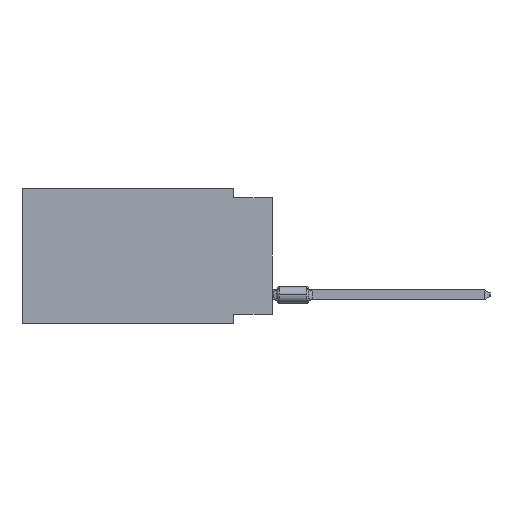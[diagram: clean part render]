
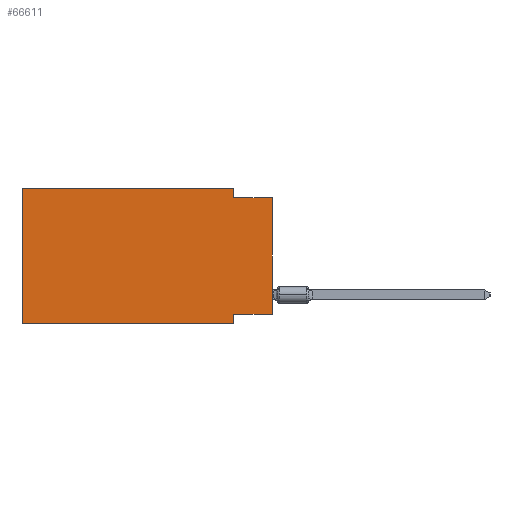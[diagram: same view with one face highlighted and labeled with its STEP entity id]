
A CAD part, left-side view. The second image highlights one B-rep face of the part: STEP entity #66611.
In plain terms, the highlighted planar face has unit normal (-1, 0, 0).
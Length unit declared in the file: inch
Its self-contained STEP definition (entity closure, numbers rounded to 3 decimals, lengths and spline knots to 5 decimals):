
#1990 = ORIENTED_EDGE ( 'NONE', *, *, #16436, .F. ) ;
#2873 = VERTEX_POINT ( 'NONE', #19491 ) ;
#4245 = LINE ( 'NONE', #48958, #18061 ) ;
#5414 = LINE ( 'NONE', #41989, #42734 ) ;
#5674 = CARTESIAN_POINT ( 'NONE',  ( 0., 0.1, -0.025 ) ) ;
#6859 = CARTESIAN_POINT ( 'NONE',  ( 0., 0.1, 0. ) ) ;
#7140 = VERTEX_POINT ( 'NONE', #83503 ) ;
#9085 = ORIENTED_EDGE ( 'NONE', *, *, #21617, .F. ) ;
#9833 = DIRECTION ( 'NONE',  ( 0., 1., 0. ) ) ;
#13986 = DIRECTION ( 'NONE',  ( 1., 0., 0. ) ) ;
#14688 = ORIENTED_EDGE ( 'NONE', *, *, #93546, .T. ) ;
#14752 = VERTEX_POINT ( 'NONE', #37182 ) ;
#15377 = LINE ( 'NONE', #66838, #82319 ) ;
#15677 = CARTESIAN_POINT ( 'NONE',  ( 0., 0., 0. ) ) ;
#16152 = DIRECTION ( 'NONE',  ( 0., 0., 1. ) ) ;
#16298 = VERTEX_POINT ( 'NONE', #43787 ) ;
#16436 = EDGE_CURVE ( 'NONE', #61065, #7140, #15377, .T. ) ;
#18061 = VECTOR ( 'NONE', #71080, 39.37008 ) ;
#19491 = CARTESIAN_POINT ( 'NONE',  ( 0., 0.1, -0.325 ) ) ;
#20256 = VECTOR ( 'NONE', #64571, 39.37008 ) ;
#21617 = EDGE_CURVE ( 'NONE', #7140, #92543, #91471, .T. ) ;
#22892 = LINE ( 'NONE', #15677, #34242 ) ;
#23430 = ORIENTED_EDGE ( 'NONE', *, *, #23758, .F. ) ;
#23758 = EDGE_CURVE ( 'NONE', #2873, #38565, #5414, .T. ) ;
#24232 = VECTOR ( 'NONE', #55381, 39.37008 ) ;
#25238 = LINE ( 'NONE', #89677, #42904 ) ;
#25363 = LINE ( 'NONE', #68623, #52701 ) ;
#29501 = EDGE_CURVE ( 'NONE', #92543, #34889, #35250, .T. ) ;
#34242 = VECTOR ( 'NONE', #16152, 39.37008 ) ;
#34720 = EDGE_CURVE ( 'NONE', #61065, #38565, #4245, .T. ) ;
#34889 = VERTEX_POINT ( 'NONE', #5674 ) ;
#34916 = ORIENTED_EDGE ( 'NONE', *, *, #93664, .F. ) ;
#35250 = LINE ( 'NONE', #6859, #20256 ) ;
#37182 = CARTESIAN_POINT ( 'NONE',  ( 0., 0., -0.325 ) ) ;
#38341 = ORIENTED_EDGE ( 'NONE', *, *, #38486, .F. ) ;
#38486 = EDGE_CURVE ( 'NONE', #14752, #2873, #25238, .T. ) ;
#38565 = VERTEX_POINT ( 'NONE', #92508 ) ;
#41989 = CARTESIAN_POINT ( 'NONE',  ( 0., 0.1, -0.35 ) ) ;
#42734 = VECTOR ( 'NONE', #71293, 39.37008 ) ;
#42904 = VECTOR ( 'NONE', #9833, 39.37008 ) ;
#43349 = DIRECTION ( 'NONE',  ( 0., 0., -1. ) ) ;
#43787 = CARTESIAN_POINT ( 'NONE',  ( 0., 0., -0.025 ) ) ;
#45525 = CARTESIAN_POINT ( 'NONE',  ( 0., 0.1, 0. ) ) ;
#48652 = CARTESIAN_POINT ( 'NONE',  ( 0., 0.645, 0. ) ) ;
#48958 = CARTESIAN_POINT ( 'NONE',  ( 0., 0.645, -0.35 ) ) ;
#52701 = VECTOR ( 'NONE', #90287, 39.37008 ) ;
#55381 = DIRECTION ( 'NONE',  ( 0., -1., 0. ) ) ;
#56013 = CARTESIAN_POINT ( 'NONE',  ( 0., 0.645, -0.35 ) ) ;
#59026 = EDGE_LOOP ( 'NONE', ( #14688, #34916, #84128, #9085, #1990, #85969, #23430, #38341 ) ) ;
#61065 = VERTEX_POINT ( 'NONE', #56013 ) ;
#64571 = DIRECTION ( 'NONE',  ( 0., 0., -1. ) ) ;
#65890 = DIRECTION ( 'NONE',  ( 0., 0., 1. ) ) ;
#66611 = ADVANCED_FACE ( 'NONE', ( #73586 ), #73121, .F. ) ;
#66838 = CARTESIAN_POINT ( 'NONE',  ( 0., 0.645, 0. ) ) ;
#68424 = AXIS2_PLACEMENT_3D ( 'NONE', #86619, #13986, #43349 ) ;
#68623 = CARTESIAN_POINT ( 'NONE',  ( 0., 0., -0.025 ) ) ;
#71080 = DIRECTION ( 'NONE',  ( 0., -1., 0. ) ) ;
#71293 = DIRECTION ( 'NONE',  ( 0., 0., -1. ) ) ;
#73121 = PLANE ( 'NONE',  #68424 ) ;
#73586 = FACE_OUTER_BOUND ( 'NONE', #59026, .T. ) ;
#82319 = VECTOR ( 'NONE', #65890, 39.37008 ) ;
#83503 = CARTESIAN_POINT ( 'NONE',  ( 0., 0.645, 0. ) ) ;
#84128 = ORIENTED_EDGE ( 'NONE', *, *, #29501, .F. ) ;
#85969 = ORIENTED_EDGE ( 'NONE', *, *, #34720, .T. ) ;
#86619 = CARTESIAN_POINT ( 'NONE',  ( 0., 0.645, 0. ) ) ;
#89677 = CARTESIAN_POINT ( 'NONE',  ( 0., 0., -0.325 ) ) ;
#90287 = DIRECTION ( 'NONE',  ( 0., -1., 0. ) ) ;
#91471 = LINE ( 'NONE', #48652, #24232 ) ;
#92508 = CARTESIAN_POINT ( 'NONE',  ( 0., 0.1, -0.35 ) ) ;
#92543 = VERTEX_POINT ( 'NONE', #45525 ) ;
#93546 = EDGE_CURVE ( 'NONE', #14752, #16298, #22892, .T. ) ;
#93664 = EDGE_CURVE ( 'NONE', #34889, #16298, #25363, .T. ) ;
